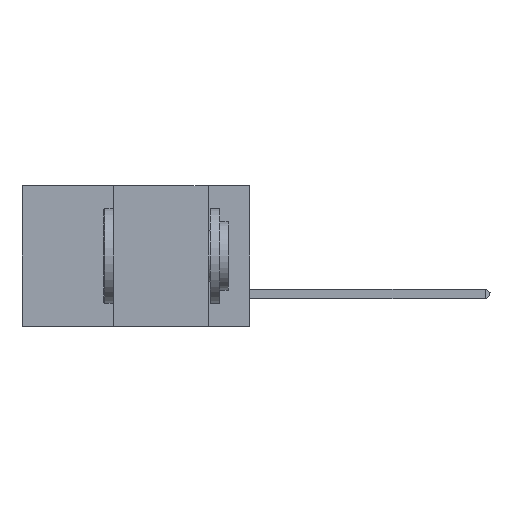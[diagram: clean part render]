
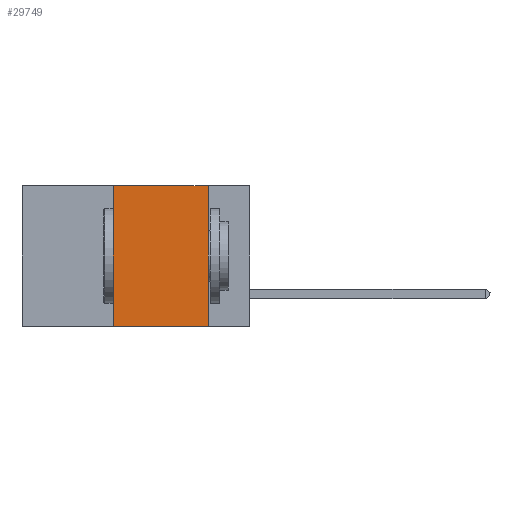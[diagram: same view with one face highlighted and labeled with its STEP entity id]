
A CAD part, left-side view. The second image highlights one B-rep face of the part: STEP entity #29749.
In plain terms, the highlighted planar face has unit normal (-1, 0, 0).
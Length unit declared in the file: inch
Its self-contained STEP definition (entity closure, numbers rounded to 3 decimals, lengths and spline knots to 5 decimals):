
#2539 = VECTOR ( 'NONE', #6625, 39.37008 ) ;
#2728 = CARTESIAN_POINT ( 'NONE',  ( 0., 0.36, 0. ) ) ;
#2993 = EDGE_LOOP ( 'NONE', ( #34546, #5590, #48291, #24457 ) ) ;
#5590 = ORIENTED_EDGE ( 'NONE', *, *, #39696, .F. ) ;
#6625 = DIRECTION ( 'NONE',  ( 0., -1., 0. ) ) ;
#7838 = VERTEX_POINT ( 'NONE', #2728 ) ;
#10394 = VECTOR ( 'NONE', #45175, 39.37008 ) ;
#12927 = VERTEX_POINT ( 'NONE', #33018 ) ;
#16742 = VERTEX_POINT ( 'NONE', #35934 ) ;
#17545 = LINE ( 'NONE', #39859, #2539 ) ;
#20166 = EDGE_CURVE ( 'NONE', #16742, #12927, #21859, .T. ) ;
#21859 = LINE ( 'NONE', #44831, #10394 ) ;
#21929 = PLANE ( 'NONE',  #48783 ) ;
#22193 = DIRECTION ( 'NONE',  ( 0., 0., -1. ) ) ;
#22896 = CARTESIAN_POINT ( 'NONE',  ( 0., 0.6, 0. ) ) ;
#24457 = ORIENTED_EDGE ( 'NONE', *, *, #20166, .T. ) ;
#24772 = VERTEX_POINT ( 'NONE', #40217 ) ;
#25506 = EDGE_CURVE ( 'NONE', #16742, #7838, #29698, .T. ) ;
#29698 = LINE ( 'NONE', #41078, #36185 ) ;
#29749 = ADVANCED_FACE ( 'NONE', ( #42463 ), #21929, .F. ) ;
#29786 = CARTESIAN_POINT ( 'NONE',  ( 0., 0.11, 0. ) ) ;
#30501 = VECTOR ( 'NONE', #22193, 39.37008 ) ;
#33018 = CARTESIAN_POINT ( 'NONE',  ( 0., 0.11, -0.37 ) ) ;
#34173 = DIRECTION ( 'NONE',  ( 0., 0., -1. ) ) ;
#34546 = ORIENTED_EDGE ( 'NONE', *, *, #36937, .F. ) ;
#35934 = CARTESIAN_POINT ( 'NONE',  ( 0., 0.36, -0.37 ) ) ;
#36185 = VECTOR ( 'NONE', #45069, 39.37008 ) ;
#36937 = EDGE_CURVE ( 'NONE', #24772, #12927, #45441, .T. ) ;
#39696 = EDGE_CURVE ( 'NONE', #7838, #24772, #17545, .T. ) ;
#39859 = CARTESIAN_POINT ( 'NONE',  ( 0., 0.6, 0. ) ) ;
#40217 = CARTESIAN_POINT ( 'NONE',  ( 0., 0.11, 0. ) ) ;
#41078 = CARTESIAN_POINT ( 'NONE',  ( 0., 0.36, 0. ) ) ;
#42205 = DIRECTION ( 'NONE',  ( 1., 0., 0. ) ) ;
#42463 = FACE_OUTER_BOUND ( 'NONE', #2993, .T. ) ;
#44831 = CARTESIAN_POINT ( 'NONE',  ( 0., 0.6, -0.37 ) ) ;
#45069 = DIRECTION ( 'NONE',  ( 0., 0., 1. ) ) ;
#45175 = DIRECTION ( 'NONE',  ( 0., -1., 0. ) ) ;
#45441 = LINE ( 'NONE', #29786, #30501 ) ;
#48291 = ORIENTED_EDGE ( 'NONE', *, *, #25506, .F. ) ;
#48783 = AXIS2_PLACEMENT_3D ( 'NONE', #22896, #42205, #34173 ) ;
